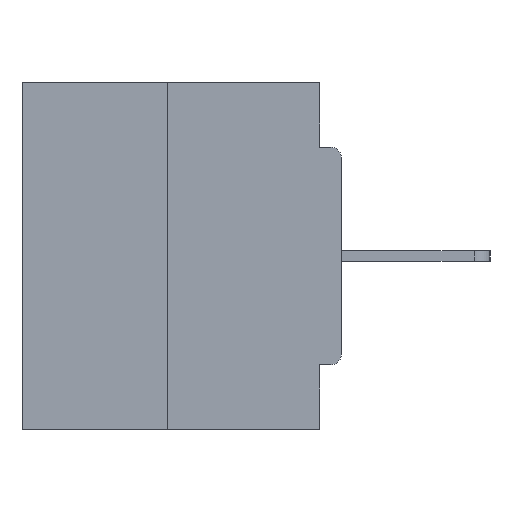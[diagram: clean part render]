
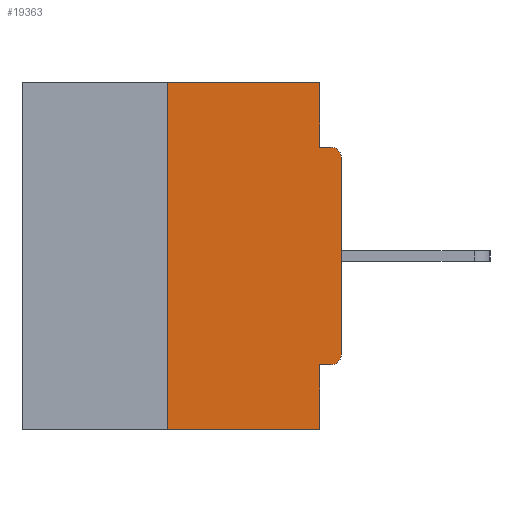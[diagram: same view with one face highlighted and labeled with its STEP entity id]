
A CAD part, left-side view. The second image highlights one B-rep face of the part: STEP entity #19363.
In plain terms, the highlighted planar face has unit normal (-1, 0, 0).
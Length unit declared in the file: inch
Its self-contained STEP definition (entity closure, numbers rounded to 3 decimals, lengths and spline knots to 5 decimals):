
#782 = AXIS2_PLACEMENT_3D ( 'NONE', #27276, #19092, #13497 ) ;
#1631 = EDGE_CURVE ( 'NONE', #10028, #21672, #8266, .T. ) ;
#1723 = VECTOR ( 'NONE', #29541, 39.37008 ) ;
#1734 = ORIENTED_EDGE ( 'NONE', *, *, #1631, .F. ) ;
#2644 = CARTESIAN_POINT ( 'NONE',  ( 0., 0.46, 0. ) ) ;
#2889 = DIRECTION ( 'NONE',  ( 0., 0., -1. ) ) ;
#3286 = DIRECTION ( 'NONE',  ( 0., 0., 1. ) ) ;
#4005 = CARTESIAN_POINT ( 'NONE',  ( 0., 0.031, -0.5 ) ) ;
#4076 = EDGE_CURVE ( 'NONE', #10968, #33649, #33672, .T. ) ;
#5171 = FACE_OUTER_BOUND ( 'NONE', #24938, .T. ) ;
#5782 = DIRECTION ( 'NONE',  ( 0., 0., -1. ) ) ;
#6400 = CARTESIAN_POINT ( 'NONE',  ( 0., 0.031, 0. ) ) ;
#7198 = VECTOR ( 'NONE', #33501, 39.37008 ) ;
#7217 = CARTESIAN_POINT ( 'NONE',  ( 0., 0., -0.1085 ) ) ;
#7787 = EDGE_CURVE ( 'NONE', #20609, #30621, #30762, .T. ) ;
#7965 = LINE ( 'NONE', #9996, #1723 ) ;
#8266 = LINE ( 'NONE', #2644, #19479 ) ;
#8517 = CARTESIAN_POINT ( 'NONE',  ( 0., 0.015, -0.1085 ) ) ;
#9370 = VERTEX_POINT ( 'NONE', #12929 ) ;
#9420 = CIRCLE ( 'NONE', #21468, 0.015 ) ;
#9438 = ORIENTED_EDGE ( 'NONE', *, *, #7787, .F. ) ;
#9996 = CARTESIAN_POINT ( 'NONE',  ( 0., 0., 0. ) ) ;
#10028 = VERTEX_POINT ( 'NONE', #29733 ) ;
#10153 = ORIENTED_EDGE ( 'NONE', *, *, #11885, .F. ) ;
#10309 = CARTESIAN_POINT ( 'NONE',  ( 0., 0.031, -0.5 ) ) ;
#10416 = EDGE_CURVE ( 'NONE', #20609, #9370, #19851, .T. ) ;
#10456 = VECTOR ( 'NONE', #13362, 39.37008 ) ;
#10968 = VERTEX_POINT ( 'NONE', #12178 ) ;
#11885 = EDGE_CURVE ( 'NONE', #20900, #20774, #16994, .T. ) ;
#12178 = CARTESIAN_POINT ( 'NONE',  ( 0., 0.25, -0.5 ) ) ;
#12829 = LINE ( 'NONE', #10309, #10456 ) ;
#12841 = VECTOR ( 'NONE', #20408, 39.37008 ) ;
#12929 = CARTESIAN_POINT ( 'NONE',  ( 0., 0., -0.3915 ) ) ;
#13250 = ORIENTED_EDGE ( 'NONE', *, *, #27543, .F. ) ;
#13362 = DIRECTION ( 'NONE',  ( 0., 0., -1. ) ) ;
#13497 = DIRECTION ( 'NONE',  ( 0., 0., -1. ) ) ;
#13514 = EDGE_CURVE ( 'NONE', #25033, #20774, #9420, .T. ) ;
#13523 = DIRECTION ( 'NONE',  ( 0., -1., 0. ) ) ;
#14280 = CARTESIAN_POINT ( 'NONE',  ( 0., 0., -0.4065 ) ) ;
#14577 = ORIENTED_EDGE ( 'NONE', *, *, #16616, .F. ) ;
#15434 = ORIENTED_EDGE ( 'NONE', *, *, #4076, .T. ) ;
#16201 = PLANE ( 'NONE',  #782 ) ;
#16616 = EDGE_CURVE ( 'NONE', #10968, #10028, #30841, .T. ) ;
#16803 = CARTESIAN_POINT ( 'NONE',  ( 0., 0., -0.0935 ) ) ;
#16994 = LINE ( 'NONE', #16803, #17044 ) ;
#17024 = LINE ( 'NONE', #27570, #30100 ) ;
#17044 = VECTOR ( 'NONE', #22971, 39.37008 ) ;
#19092 = DIRECTION ( 'NONE',  ( 1., 0., 0. ) ) ;
#19363 = ADVANCED_FACE ( 'NONE', ( #5171 ), #16201, .F. ) ;
#19479 = VECTOR ( 'NONE', #13523, 39.37008 ) ;
#19535 = DIRECTION ( 'NONE',  ( -1., 0., 0. ) ) ;
#19851 = CIRCLE ( 'NONE', #23941, 0.015 ) ;
#20408 = DIRECTION ( 'NONE',  ( 0., 1., 0. ) ) ;
#20609 = VERTEX_POINT ( 'NONE', #29701 ) ;
#20774 = VERTEX_POINT ( 'NONE', #33354 ) ;
#20900 = VERTEX_POINT ( 'NONE', #23691 ) ;
#21095 = VECTOR ( 'NONE', #3286, 39.37008 ) ;
#21176 = ORIENTED_EDGE ( 'NONE', *, *, #25953, .F. ) ;
#21343 = DIRECTION ( 'NONE',  ( 0., 0., -1. ) ) ;
#21468 = AXIS2_PLACEMENT_3D ( 'NONE', #8517, #19535, #5782 ) ;
#21672 = VERTEX_POINT ( 'NONE', #6400 ) ;
#22971 = DIRECTION ( 'NONE',  ( 0., -1., 0. ) ) ;
#23691 = CARTESIAN_POINT ( 'NONE',  ( 0., 0.031, -0.0935 ) ) ;
#23941 = AXIS2_PLACEMENT_3D ( 'NONE', #35533, #27335, #21343 ) ;
#24483 = ORIENTED_EDGE ( 'NONE', *, *, #10416, .T. ) ;
#24938 = EDGE_LOOP ( 'NONE', ( #1734, #14577, #15434, #13250, #9438, #24483, #31935, #25918, #10153, #21176 ) ) ;
#25033 = VERTEX_POINT ( 'NONE', #7217 ) ;
#25410 = CARTESIAN_POINT ( 'NONE',  ( 0., 0.25, 0. ) ) ;
#25823 = EDGE_CURVE ( 'NONE', #9370, #25033, #7965, .T. ) ;
#25918 = ORIENTED_EDGE ( 'NONE', *, *, #13514, .T. ) ;
#25953 = EDGE_CURVE ( 'NONE', #21672, #20900, #17024, .T. ) ;
#26213 = CARTESIAN_POINT ( 'NONE',  ( 0., 0.031, -0.4065 ) ) ;
#27276 = CARTESIAN_POINT ( 'NONE',  ( 0., 0.46, 0. ) ) ;
#27335 = DIRECTION ( 'NONE',  ( -1., 0., 0. ) ) ;
#27543 = EDGE_CURVE ( 'NONE', #30621, #33649, #12829, .T. ) ;
#27570 = CARTESIAN_POINT ( 'NONE',  ( 0., 0.031, 0. ) ) ;
#29541 = DIRECTION ( 'NONE',  ( 0., 0., 1. ) ) ;
#29701 = CARTESIAN_POINT ( 'NONE',  ( 0., 0.015, -0.4065 ) ) ;
#29733 = CARTESIAN_POINT ( 'NONE',  ( 0., 0.25, 0. ) ) ;
#30100 = VECTOR ( 'NONE', #2889, 39.37008 ) ;
#30621 = VERTEX_POINT ( 'NONE', #26213 ) ;
#30747 = CARTESIAN_POINT ( 'NONE',  ( 0., 0.46, -0.5 ) ) ;
#30762 = LINE ( 'NONE', #14280, #12841 ) ;
#30841 = LINE ( 'NONE', #25410, #21095 ) ;
#31935 = ORIENTED_EDGE ( 'NONE', *, *, #25823, .T. ) ;
#33354 = CARTESIAN_POINT ( 'NONE',  ( 0., 0.015, -0.0935 ) ) ;
#33501 = DIRECTION ( 'NONE',  ( 0., -1., 0. ) ) ;
#33649 = VERTEX_POINT ( 'NONE', #4005 ) ;
#33672 = LINE ( 'NONE', #30747, #7198 ) ;
#35533 = CARTESIAN_POINT ( 'NONE',  ( 0., 0.015, -0.3915 ) ) ;
